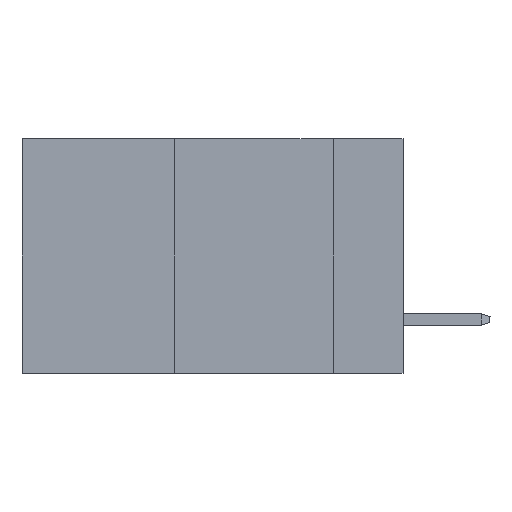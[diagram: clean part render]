
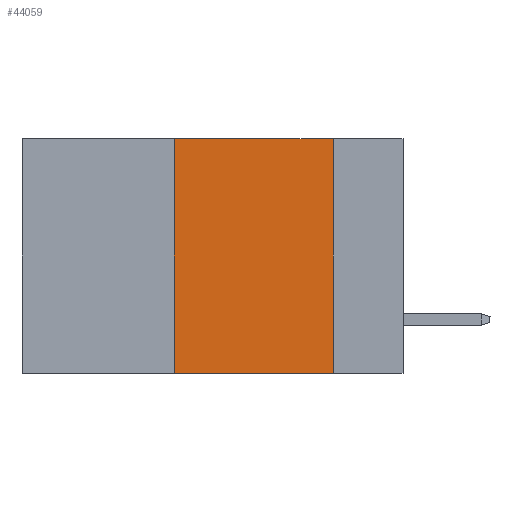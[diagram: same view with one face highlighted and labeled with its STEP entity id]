
A CAD part, left-side view. The second image highlights one B-rep face of the part: STEP entity #44059.
In plain terms, the highlighted planar face has unit normal (-1, 0, 0).
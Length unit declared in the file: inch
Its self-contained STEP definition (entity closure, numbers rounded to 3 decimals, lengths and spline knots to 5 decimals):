
#851 = EDGE_CURVE ( 'NONE', #27503, #17093, #11749, .T. ) ;
#3814 = CARTESIAN_POINT ( 'NONE',  ( 0., 0.11, 0. ) ) ;
#4969 = CARTESIAN_POINT ( 'NONE',  ( 0., 0.36, -0.37 ) ) ;
#5449 = VECTOR ( 'NONE', #17182, 39.37008 ) ;
#5982 = CARTESIAN_POINT ( 'NONE',  ( 0., 0.36, 0. ) ) ;
#7833 = DIRECTION ( 'NONE',  ( 0., 0., -1. ) ) ;
#11749 = LINE ( 'NONE', #34794, #26569 ) ;
#12769 = LINE ( 'NONE', #18063, #5449 ) ;
#13096 = CARTESIAN_POINT ( 'NONE',  ( 0., 0.11, -0.37 ) ) ;
#14015 = VERTEX_POINT ( 'NONE', #4969 ) ;
#16835 = ORIENTED_EDGE ( 'NONE', *, *, #17420, .F. ) ;
#16930 = ORIENTED_EDGE ( 'NONE', *, *, #36913, .T. ) ;
#17093 = VERTEX_POINT ( 'NONE', #27260 ) ;
#17182 = DIRECTION ( 'NONE',  ( 0., -1., 0. ) ) ;
#17420 = EDGE_CURVE ( 'NONE', #14015, #27503, #22940, .T. ) ;
#18063 = CARTESIAN_POINT ( 'NONE',  ( 0., 0.6, -0.37 ) ) ;
#18224 = ORIENTED_EDGE ( 'NONE', *, *, #851, .F. ) ;
#21304 = EDGE_LOOP ( 'NONE', ( #35032, #18224, #16835, #16930 ) ) ;
#21558 = DIRECTION ( 'NONE',  ( 0., -1., 0. ) ) ;
#21812 = CARTESIAN_POINT ( 'NONE',  ( 0., 0.6, 0. ) ) ;
#22940 = LINE ( 'NONE', #5982, #24659 ) ;
#24659 = VECTOR ( 'NONE', #33478, 39.37008 ) ;
#25161 = VECTOR ( 'NONE', #7833, 39.37008 ) ;
#25181 = FACE_OUTER_BOUND ( 'NONE', #21304, .T. ) ;
#26569 = VECTOR ( 'NONE', #21558, 39.37008 ) ;
#27260 = CARTESIAN_POINT ( 'NONE',  ( 0., 0.11, 0. ) ) ;
#27503 = VERTEX_POINT ( 'NONE', #34611 ) ;
#29000 = DIRECTION ( 'NONE',  ( 1., 0., 0. ) ) ;
#29740 = VERTEX_POINT ( 'NONE', #13096 ) ;
#33478 = DIRECTION ( 'NONE',  ( 0., 0., 1. ) ) ;
#34611 = CARTESIAN_POINT ( 'NONE',  ( 0., 0.36, 0. ) ) ;
#34794 = CARTESIAN_POINT ( 'NONE',  ( 0., 0.6, 0. ) ) ;
#35032 = ORIENTED_EDGE ( 'NONE', *, *, #38276, .F. ) ;
#35317 = LINE ( 'NONE', #3814, #25161 ) ;
#35436 = AXIS2_PLACEMENT_3D ( 'NONE', #21812, #29000, #35475 ) ;
#35475 = DIRECTION ( 'NONE',  ( 0., 0., -1. ) ) ;
#36913 = EDGE_CURVE ( 'NONE', #14015, #29740, #12769, .T. ) ;
#38276 = EDGE_CURVE ( 'NONE', #17093, #29740, #35317, .T. ) ;
#38824 = PLANE ( 'NONE',  #35436 ) ;
#44059 = ADVANCED_FACE ( 'NONE', ( #25181 ), #38824, .F. ) ;
